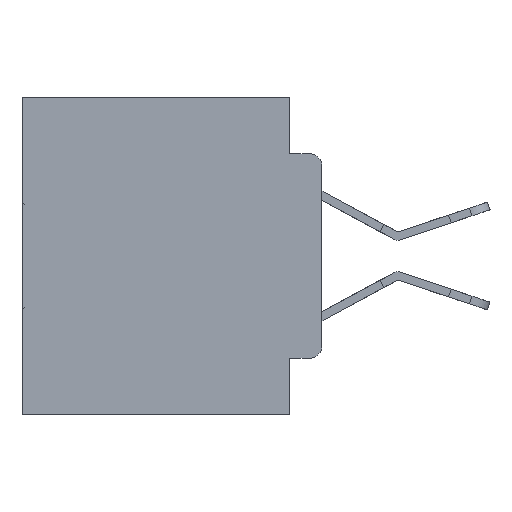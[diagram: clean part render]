
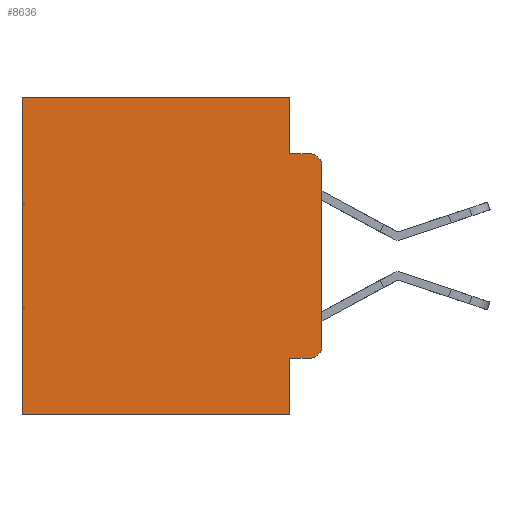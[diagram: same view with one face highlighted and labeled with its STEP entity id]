
A CAD part, left-side view. The second image highlights one B-rep face of the part: STEP entity #8636.
In plain terms, the highlighted planar face has unit normal (-1, 0, 0).
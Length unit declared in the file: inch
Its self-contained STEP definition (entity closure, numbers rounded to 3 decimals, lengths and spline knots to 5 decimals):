
#102 = CIRCLE ( 'NONE', #1020, 0.02 ) ;
#494 = VERTEX_POINT ( 'NONE', #30365 ) ;
#632 = CARTESIAN_POINT ( 'NONE',  ( 0.298, 0.473, 0. ) ) ;
#1000 = ORIENTED_EDGE ( 'NONE', *, *, #29893, .T. ) ;
#1020 = AXIS2_PLACEMENT_3D ( 'NONE', #3645, #21868, #6290 ) ;
#1072 = VECTOR ( 'NONE', #14045, 39.37008 ) ;
#2168 = ORIENTED_EDGE ( 'NONE', *, *, #30517, .T. ) ;
#2657 = LINE ( 'NONE', #26862, #1072 ) ;
#3645 = CARTESIAN_POINT ( 'NONE',  ( 0.298, 0.02, -0.1085 ) ) ;
#4844 = CARTESIAN_POINT ( 'NONE',  ( 0.298, 0.051, -0.5 ) ) ;
#5214 = VECTOR ( 'NONE', #31833, 39.37008 ) ;
#6175 = VERTEX_POINT ( 'NONE', #17321 ) ;
#6290 = DIRECTION ( 'NONE',  ( 0., 0., -1. ) ) ;
#6479 = LINE ( 'NONE', #27299, #33010 ) ;
#7493 = ORIENTED_EDGE ( 'NONE', *, *, #16367, .T. ) ;
#8636 = ADVANCED_FACE ( 'NONE', ( #10344 ), #29397, .F. ) ;
#8684 = CARTESIAN_POINT ( 'NONE',  ( 0.298, 0., 0. ) ) ;
#9197 = DIRECTION ( 'NONE',  ( 0., -1., 0. ) ) ;
#9367 = DIRECTION ( 'NONE',  ( 0., 0., -1. ) ) ;
#9385 = EDGE_CURVE ( 'NONE', #22306, #12783, #16017, .T. ) ;
#9426 = CARTESIAN_POINT ( 'NONE',  ( 0.298, 0.051, -0.0885 ) ) ;
#9517 = ORIENTED_EDGE ( 'NONE', *, *, #11799, .F. ) ;
#9568 = CARTESIAN_POINT ( 'NONE',  ( 0.298, 0.02, -0.4115 ) ) ;
#10209 = VECTOR ( 'NONE', #9197, 39.37008 ) ;
#10344 = FACE_OUTER_BOUND ( 'NONE', #25611, .T. ) ;
#10657 = CARTESIAN_POINT ( 'NONE',  ( 0.298, 0.051, 0. ) ) ;
#10963 = DIRECTION ( 'NONE',  ( 0., 0., -1. ) ) ;
#11687 = DIRECTION ( 'NONE',  ( -1., 0., 0. ) ) ;
#11799 = EDGE_CURVE ( 'NONE', #32161, #494, #32230, .T. ) ;
#11991 = ORIENTED_EDGE ( 'NONE', *, *, #23531, .F. ) ;
#12413 = VERTEX_POINT ( 'NONE', #29751 ) ;
#12655 = EDGE_CURVE ( 'NONE', #12413, #6175, #13353, .T. ) ;
#12783 = VERTEX_POINT ( 'NONE', #23525 ) ;
#13210 = VERTEX_POINT ( 'NONE', #9568 ) ;
#13353 = LINE ( 'NONE', #15299, #31383 ) ;
#14045 = DIRECTION ( 'NONE',  ( 0., 0., -1. ) ) ;
#14103 = VERTEX_POINT ( 'NONE', #632 ) ;
#14824 = ORIENTED_EDGE ( 'NONE', *, *, #12655, .F. ) ;
#15299 = CARTESIAN_POINT ( 'NONE',  ( 0.298, 0., 0. ) ) ;
#16017 = LINE ( 'NONE', #31006, #28782 ) ;
#16367 = EDGE_CURVE ( 'NONE', #24554, #14103, #32614, .T. ) ;
#17321 = CARTESIAN_POINT ( 'NONE',  ( 0.298, 0., -0.3915 ) ) ;
#18254 = CARTESIAN_POINT ( 'NONE',  ( 0.298, 0.051, -0.4115 ) ) ;
#18663 = VECTOR ( 'NONE', #30021, 39.37008 ) ;
#20548 = DIRECTION ( 'NONE',  ( 0., 1., 0. ) ) ;
#21641 = CARTESIAN_POINT ( 'NONE',  ( 0.298, 0., 0. ) ) ;
#21868 = DIRECTION ( 'NONE',  ( -1., 0., 0. ) ) ;
#22172 = CARTESIAN_POINT ( 'NONE',  ( 0.298, 0.051, -0.4115 ) ) ;
#22306 = VERTEX_POINT ( 'NONE', #4844 ) ;
#22526 = ORIENTED_EDGE ( 'NONE', *, *, #26451, .T. ) ;
#22825 = CARTESIAN_POINT ( 'NONE',  ( 0.298, 0.051, -0.0885 ) ) ;
#22935 = ORIENTED_EDGE ( 'NONE', *, *, #9385, .F. ) ;
#23436 = EDGE_CURVE ( 'NONE', #27384, #22306, #31736, .T. ) ;
#23525 = CARTESIAN_POINT ( 'NONE',  ( 0.298, 0.473, -0.5 ) ) ;
#23531 = EDGE_CURVE ( 'NONE', #24554, #32161, #2657, .T. ) ;
#23854 = CARTESIAN_POINT ( 'NONE',  ( 0.298, 0.051, 0. ) ) ;
#24533 = ORIENTED_EDGE ( 'NONE', *, *, #23436, .F. ) ;
#24554 = VERTEX_POINT ( 'NONE', #10657 ) ;
#24800 = LINE ( 'NONE', #22172, #10209 ) ;
#25139 = CIRCLE ( 'NONE', #32606, 0.02 ) ;
#25306 = ORIENTED_EDGE ( 'NONE', *, *, #29231, .T. ) ;
#25611 = EDGE_LOOP ( 'NONE', ( #14824, #22526, #9517, #11991, #7493, #2168, #22935, #24533, #25306, #1000 ) ) ;
#26451 = EDGE_CURVE ( 'NONE', #12413, #494, #102, .T. ) ;
#26862 = CARTESIAN_POINT ( 'NONE',  ( 0.298, 0.051, 0. ) ) ;
#27117 = CARTESIAN_POINT ( 'NONE',  ( 0.298, 0.02, -0.3915 ) ) ;
#27299 = CARTESIAN_POINT ( 'NONE',  ( 0.298, 0.473, 0. ) ) ;
#27384 = VERTEX_POINT ( 'NONE', #18254 ) ;
#27696 = AXIS2_PLACEMENT_3D ( 'NONE', #8684, #27741, #31943 ) ;
#27741 = DIRECTION ( 'NONE',  ( 1., 0., 0. ) ) ;
#28782 = VECTOR ( 'NONE', #20548, 39.37008 ) ;
#29231 = EDGE_CURVE ( 'NONE', #27384, #13210, #24800, .T. ) ;
#29397 = PLANE ( 'NONE',  #27696 ) ;
#29653 = DIRECTION ( 'NONE',  ( 0., 0., -1. ) ) ;
#29751 = CARTESIAN_POINT ( 'NONE',  ( 0.298, 0., -0.1085 ) ) ;
#29893 = EDGE_CURVE ( 'NONE', #13210, #6175, #25139, .T. ) ;
#30021 = DIRECTION ( 'NONE',  ( 0., -1., 0. ) ) ;
#30365 = CARTESIAN_POINT ( 'NONE',  ( 0.298, 0.02, -0.0885 ) ) ;
#30517 = EDGE_CURVE ( 'NONE', #14103, #12783, #6479, .T. ) ;
#30632 = DIRECTION ( 'NONE',  ( 0., 0., -1. ) ) ;
#31006 = CARTESIAN_POINT ( 'NONE',  ( 0.298, 0., -0.5 ) ) ;
#31383 = VECTOR ( 'NONE', #30632, 39.37008 ) ;
#31736 = LINE ( 'NONE', #23854, #32539 ) ;
#31833 = DIRECTION ( 'NONE',  ( 0., 1., 0. ) ) ;
#31943 = DIRECTION ( 'NONE',  ( 0., 0., -1. ) ) ;
#32161 = VERTEX_POINT ( 'NONE', #22825 ) ;
#32230 = LINE ( 'NONE', #9426, #18663 ) ;
#32539 = VECTOR ( 'NONE', #10963, 39.37008 ) ;
#32606 = AXIS2_PLACEMENT_3D ( 'NONE', #27117, #11687, #29653 ) ;
#32614 = LINE ( 'NONE', #21641, #5214 ) ;
#33010 = VECTOR ( 'NONE', #9367, 39.37008 ) ;
